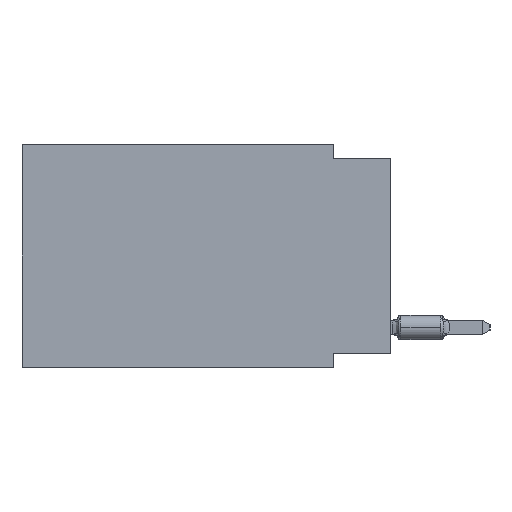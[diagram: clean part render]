
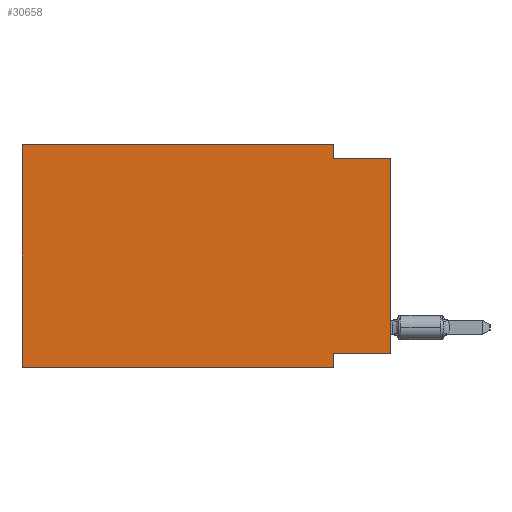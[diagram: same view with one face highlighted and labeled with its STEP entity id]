
A CAD part, left-side view. The second image highlights one B-rep face of the part: STEP entity #30658.
In plain terms, the highlighted planar face has unit normal (-1, 0, 0).
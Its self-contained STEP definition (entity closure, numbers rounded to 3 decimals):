
#244 = CARTESIAN_POINT ( 'NONE',  ( 0., 2.54, -9.271 ) ) ;
#886 = EDGE_CURVE ( 'NONE', #33675, #2308, #12503, .T. ) ;
#910 = ORIENTED_EDGE ( 'NONE', *, *, #15662, .F. ) ;
#2297 = VECTOR ( 'NONE', #15554, 1000. ) ;
#2308 = VERTEX_POINT ( 'NONE', #5113 ) ;
#2738 = CARTESIAN_POINT ( 'NONE',  ( 0., 2.54, -9.906 ) ) ;
#2801 = DIRECTION ( 'NONE',  ( 0., 0., -1. ) ) ;
#3178 = CARTESIAN_POINT ( 'NONE',  ( 0., 2.54, -9.906 ) ) ;
#4297 = DIRECTION ( 'NONE',  ( 0., 0., -1. ) ) ;
#4335 = VECTOR ( 'NONE', #13821, 1000. ) ;
#4980 = LINE ( 'NONE', #33754, #33054 ) ;
#5113 = CARTESIAN_POINT ( 'NONE',  ( 0., 2.54, 0. ) ) ;
#6549 = DIRECTION ( 'NONE',  ( 0., -1., 0. ) ) ;
#7365 = ORIENTED_EDGE ( 'NONE', *, *, #16199, .F. ) ;
#7443 = DIRECTION ( 'NONE',  ( 0., 0., -1. ) ) ;
#7492 = EDGE_CURVE ( 'NONE', #37378, #33675, #36705, .T. ) ;
#8699 = FACE_OUTER_BOUND ( 'NONE', #29460, .T. ) ;
#9289 = CARTESIAN_POINT ( 'NONE',  ( 0., 16.383, -9.906 ) ) ;
#9509 = CARTESIAN_POINT ( 'NONE',  ( 0., 0., -9.271 ) ) ;
#9521 = VECTOR ( 'NONE', #20932, 1000. ) ;
#9978 = VERTEX_POINT ( 'NONE', #2738 ) ;
#11765 = EDGE_CURVE ( 'NONE', #33057, #35784, #15911, .T. ) ;
#12053 = CARTESIAN_POINT ( 'NONE',  ( 0., 0., -0.635 ) ) ;
#12503 = LINE ( 'NONE', #29713, #13951 ) ;
#13821 = DIRECTION ( 'NONE',  ( 0., 0., 1. ) ) ;
#13951 = VECTOR ( 'NONE', #26876, 1000. ) ;
#14766 = ORIENTED_EDGE ( 'NONE', *, *, #23139, .T. ) ;
#14903 = ORIENTED_EDGE ( 'NONE', *, *, #886, .F. ) ;
#15252 = CARTESIAN_POINT ( 'NONE',  ( 0., 0., 0. ) ) ;
#15376 = ORIENTED_EDGE ( 'NONE', *, *, #15527, .T. ) ;
#15527 = EDGE_CURVE ( 'NONE', #33057, #26620, #29440, .T. ) ;
#15554 = DIRECTION ( 'NONE',  ( 0., 1., 0. ) ) ;
#15662 = EDGE_CURVE ( 'NONE', #2308, #25408, #4980, .T. ) ;
#15911 = LINE ( 'NONE', #9509, #2297 ) ;
#16199 = EDGE_CURVE ( 'NONE', #35784, #9978, #28922, .T. ) ;
#16941 = AXIS2_PLACEMENT_3D ( 'NONE', #17957, #29502, #4297 ) ;
#17957 = CARTESIAN_POINT ( 'NONE',  ( 0., 16.383, 0. ) ) ;
#18488 = CARTESIAN_POINT ( 'NONE',  ( 0., 16.383, -9.906 ) ) ;
#18666 = VECTOR ( 'NONE', #6549, 1000. ) ;
#20062 = LINE ( 'NONE', #12053, #18666 ) ;
#20195 = CARTESIAN_POINT ( 'NONE',  ( 0., 0., -9.271 ) ) ;
#20932 = DIRECTION ( 'NONE',  ( 0., 0., 1. ) ) ;
#23139 = EDGE_CURVE ( 'NONE', #37378, #9978, #35395, .T. ) ;
#23361 = ORIENTED_EDGE ( 'NONE', *, *, #29384, .F. ) ;
#25214 = VECTOR ( 'NONE', #2801, 1000. ) ;
#25408 = VERTEX_POINT ( 'NONE', #26095 ) ;
#25770 = CARTESIAN_POINT ( 'NONE',  ( 0., 0., -0.635 ) ) ;
#26095 = CARTESIAN_POINT ( 'NONE',  ( 0., 2.54, -0.635 ) ) ;
#26620 = VERTEX_POINT ( 'NONE', #25770 ) ;
#26876 = DIRECTION ( 'NONE',  ( 0., -1., 0. ) ) ;
#28922 = LINE ( 'NONE', #3178, #25214 ) ;
#29384 = EDGE_CURVE ( 'NONE', #25408, #26620, #20062, .T. ) ;
#29440 = LINE ( 'NONE', #15252, #9521 ) ;
#29460 = EDGE_LOOP ( 'NONE', ( #15376, #23361, #910, #14903, #29709, #14766, #7365, #31902 ) ) ;
#29502 = DIRECTION ( 'NONE',  ( 1., 0., 0. ) ) ;
#29709 = ORIENTED_EDGE ( 'NONE', *, *, #7492, .F. ) ;
#29713 = CARTESIAN_POINT ( 'NONE',  ( 0., 16.383, 0. ) ) ;
#30658 = ADVANCED_FACE ( 'NONE', ( #8699 ), #31780, .F. ) ;
#31780 = PLANE ( 'NONE',  #16941 ) ;
#31902 = ORIENTED_EDGE ( 'NONE', *, *, #11765, .F. ) ;
#32370 = DIRECTION ( 'NONE',  ( 0., -1., 0. ) ) ;
#33054 = VECTOR ( 'NONE', #7443, 1000. ) ;
#33057 = VERTEX_POINT ( 'NONE', #20195 ) ;
#33675 = VERTEX_POINT ( 'NONE', #33711 ) ;
#33711 = CARTESIAN_POINT ( 'NONE',  ( 0., 16.383, 0. ) ) ;
#33754 = CARTESIAN_POINT ( 'NONE',  ( 0., 2.54, 0. ) ) ;
#34263 = CARTESIAN_POINT ( 'NONE',  ( 0., 16.383, 0. ) ) ;
#34763 = VECTOR ( 'NONE', #32370, 1000. ) ;
#35395 = LINE ( 'NONE', #9289, #34763 ) ;
#35784 = VERTEX_POINT ( 'NONE', #244 ) ;
#36705 = LINE ( 'NONE', #34263, #4335 ) ;
#37378 = VERTEX_POINT ( 'NONE', #18488 ) ;
